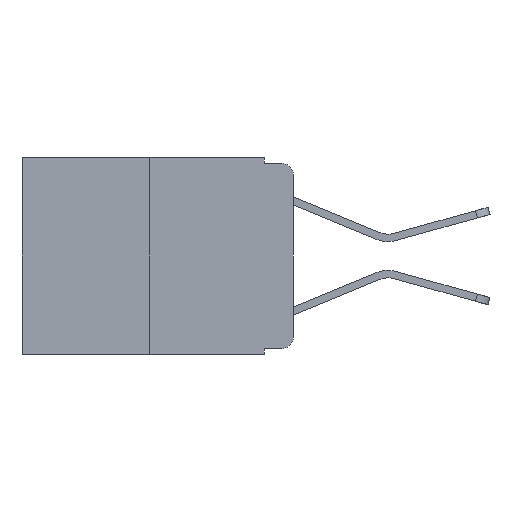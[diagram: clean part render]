
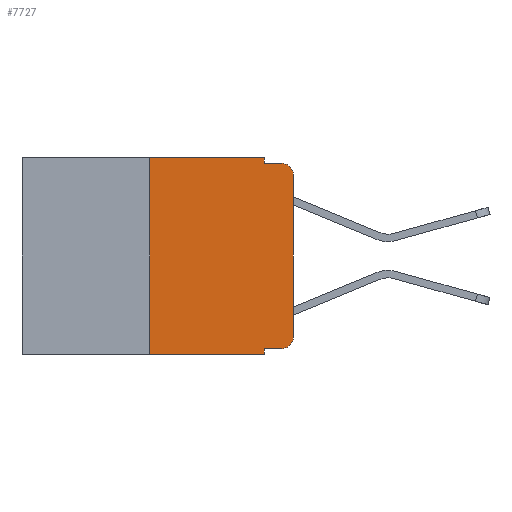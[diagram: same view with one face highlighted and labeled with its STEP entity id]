
A CAD part, left-side view. The second image highlights one B-rep face of the part: STEP entity #7727.
In plain terms, the highlighted planar face has unit normal (-1, 0, 0).
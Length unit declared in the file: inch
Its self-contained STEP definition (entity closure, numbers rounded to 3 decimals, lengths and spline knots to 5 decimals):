
#19 = VECTOR ( 'NONE', #976, 39.37008 ) ;
#182 = CARTESIAN_POINT ( 'NONE',  ( 0., 0.02, -0.333 ) ) ;
#357 = VERTEX_POINT ( 'NONE', #7337 ) ;
#463 = LINE ( 'NONE', #1915, #8980 ) ;
#518 = CARTESIAN_POINT ( 'NONE',  ( 0., 0.051, -0.343 ) ) ;
#529 = CARTESIAN_POINT ( 'NONE',  ( 0., 0.473, -0.343 ) ) ;
#762 = AXIS2_PLACEMENT_3D ( 'NONE', #8614, #8347, #8322 ) ;
#814 = DIRECTION ( 'NONE',  ( 0., 0., -1. ) ) ;
#976 = DIRECTION ( 'NONE',  ( 0., -1., 0. ) ) ;
#1372 = VECTOR ( 'NONE', #4369, 39.37008 ) ;
#1498 = DIRECTION ( 'NONE',  ( 0., -1., 0. ) ) ;
#1502 = DIRECTION ( 'NONE',  ( 0., -1., 0. ) ) ;
#1587 = AXIS2_PLACEMENT_3D ( 'NONE', #1830, #4417, #5062 ) ;
#1641 = LINE ( 'NONE', #9610, #4080 ) ;
#1738 = LINE ( 'NONE', #2721, #10632 ) ;
#1830 = CARTESIAN_POINT ( 'NONE',  ( 0., 0.02, -0.313 ) ) ;
#1857 = EDGE_CURVE ( 'NONE', #3834, #5752, #1641, .T. ) ;
#1915 = CARTESIAN_POINT ( 'NONE',  ( 0., 0.051, -0.01 ) ) ;
#2013 = VERTEX_POINT ( 'NONE', #518 ) ;
#2149 = CARTESIAN_POINT ( 'NONE',  ( 0., 0., -0.313 ) ) ;
#2237 = ORIENTED_EDGE ( 'NONE', *, *, #7887, .T. ) ;
#2522 = ORIENTED_EDGE ( 'NONE', *, *, #1857, .F. ) ;
#2638 = LINE ( 'NONE', #3623, #4421 ) ;
#2721 = CARTESIAN_POINT ( 'NONE',  ( 0., 0.25, 0. ) ) ;
#3091 = EDGE_CURVE ( 'NONE', #3539, #4905, #9363, .T. ) ;
#3094 = ORIENTED_EDGE ( 'NONE', *, *, #6997, .F. ) ;
#3133 = CARTESIAN_POINT ( 'NONE',  ( 0., 0.25, -0.343 ) ) ;
#3193 = CARTESIAN_POINT ( 'NONE',  ( 0., 0.25, 0. ) ) ;
#3401 = CARTESIAN_POINT ( 'NONE',  ( 0., 0.051, -0.333 ) ) ;
#3539 = VERTEX_POINT ( 'NONE', #6509 ) ;
#3623 = CARTESIAN_POINT ( 'NONE',  ( 0., 0.051, 0. ) ) ;
#3834 = VERTEX_POINT ( 'NONE', #3193 ) ;
#3870 = LINE ( 'NONE', #6930, #10365 ) ;
#3908 = EDGE_CURVE ( 'NONE', #4905, #10495, #9244, .T. ) ;
#3931 = VERTEX_POINT ( 'NONE', #8288 ) ;
#4080 = VECTOR ( 'NONE', #1498, 39.37008 ) ;
#4369 = DIRECTION ( 'NONE',  ( 0., 0., -1. ) ) ;
#4417 = DIRECTION ( 'NONE',  ( -1., 0., 0. ) ) ;
#4421 = VECTOR ( 'NONE', #814, 39.37008 ) ;
#4495 = ORIENTED_EDGE ( 'NONE', *, *, #5066, .T. ) ;
#4582 = ORIENTED_EDGE ( 'NONE', *, *, #8525, .F. ) ;
#4634 = LINE ( 'NONE', #6871, #1372 ) ;
#4838 = ORIENTED_EDGE ( 'NONE', *, *, #10119, .F. ) ;
#4905 = VERTEX_POINT ( 'NONE', #182 ) ;
#4960 = DIRECTION ( 'NONE',  ( -1., 0., 0. ) ) ;
#5062 = DIRECTION ( 'NONE',  ( 0., 0., -1. ) ) ;
#5066 = EDGE_CURVE ( 'NONE', #3931, #5876, #5356, .T. ) ;
#5356 = CIRCLE ( 'NONE', #6998, 0.02 ) ;
#5396 = ORIENTED_EDGE ( 'NONE', *, *, #10804, .T. ) ;
#5453 = DIRECTION ( 'NONE',  ( 0., -1., 0. ) ) ;
#5752 = VERTEX_POINT ( 'NONE', #9613 ) ;
#5876 = VERTEX_POINT ( 'NONE', #9544 ) ;
#6157 = DIRECTION ( 'NONE',  ( 0., 0., 1. ) ) ;
#6270 = VERTEX_POINT ( 'NONE', #3133 ) ;
#6501 = FACE_OUTER_BOUND ( 'NONE', #9141, .T. ) ;
#6509 = CARTESIAN_POINT ( 'NONE',  ( 0., 0.051, -0.333 ) ) ;
#6871 = CARTESIAN_POINT ( 'NONE',  ( 0., 0.051, 0. ) ) ;
#6910 = DIRECTION ( 'NONE',  ( 0., 0., 1. ) ) ;
#6930 = CARTESIAN_POINT ( 'NONE',  ( 0., 0., 0. ) ) ;
#6997 = EDGE_CURVE ( 'NONE', #6270, #3834, #1738, .T. ) ;
#6998 = AXIS2_PLACEMENT_3D ( 'NONE', #8333, #4960, #10621 ) ;
#7087 = ORIENTED_EDGE ( 'NONE', *, *, #3908, .T. ) ;
#7337 = CARTESIAN_POINT ( 'NONE',  ( 0., 0.051, -0.01 ) ) ;
#7727 = ADVANCED_FACE ( 'NONE', ( #6501 ), #8372, .F. ) ;
#7887 = EDGE_CURVE ( 'NONE', #10495, #3931, #3870, .T. ) ;
#8288 = CARTESIAN_POINT ( 'NONE',  ( 0., 0., -0.03 ) ) ;
#8322 = DIRECTION ( 'NONE',  ( 0., 0., -1. ) ) ;
#8333 = CARTESIAN_POINT ( 'NONE',  ( 0., 0.02, -0.03 ) ) ;
#8347 = DIRECTION ( 'NONE',  ( 1., 0., 0. ) ) ;
#8372 = PLANE ( 'NONE',  #762 ) ;
#8525 = EDGE_CURVE ( 'NONE', #5752, #357, #2638, .T. ) ;
#8614 = CARTESIAN_POINT ( 'NONE',  ( 0., 0.473, 0. ) ) ;
#8980 = VECTOR ( 'NONE', #5453, 39.37008 ) ;
#8989 = EDGE_CURVE ( 'NONE', #357, #5876, #463, .T. ) ;
#9141 = EDGE_LOOP ( 'NONE', ( #2237, #4495, #9722, #4582, #2522, #3094, #5396, #4838, #9264, #7087 ) ) ;
#9244 = CIRCLE ( 'NONE', #1587, 0.02 ) ;
#9264 = ORIENTED_EDGE ( 'NONE', *, *, #3091, .T. ) ;
#9363 = LINE ( 'NONE', #3401, #19 ) ;
#9544 = CARTESIAN_POINT ( 'NONE',  ( 0., 0.02, -0.01 ) ) ;
#9610 = CARTESIAN_POINT ( 'NONE',  ( 0., 0.473, 0. ) ) ;
#9613 = CARTESIAN_POINT ( 'NONE',  ( 0., 0.051, 0. ) ) ;
#9722 = ORIENTED_EDGE ( 'NONE', *, *, #8989, .F. ) ;
#10119 = EDGE_CURVE ( 'NONE', #3539, #2013, #4634, .T. ) ;
#10221 = VECTOR ( 'NONE', #1502, 39.37008 ) ;
#10365 = VECTOR ( 'NONE', #6910, 39.37008 ) ;
#10460 = LINE ( 'NONE', #529, #10221 ) ;
#10495 = VERTEX_POINT ( 'NONE', #2149 ) ;
#10621 = DIRECTION ( 'NONE',  ( 0., 0., -1. ) ) ;
#10632 = VECTOR ( 'NONE', #6157, 39.37008 ) ;
#10804 = EDGE_CURVE ( 'NONE', #6270, #2013, #10460, .T. ) ;
